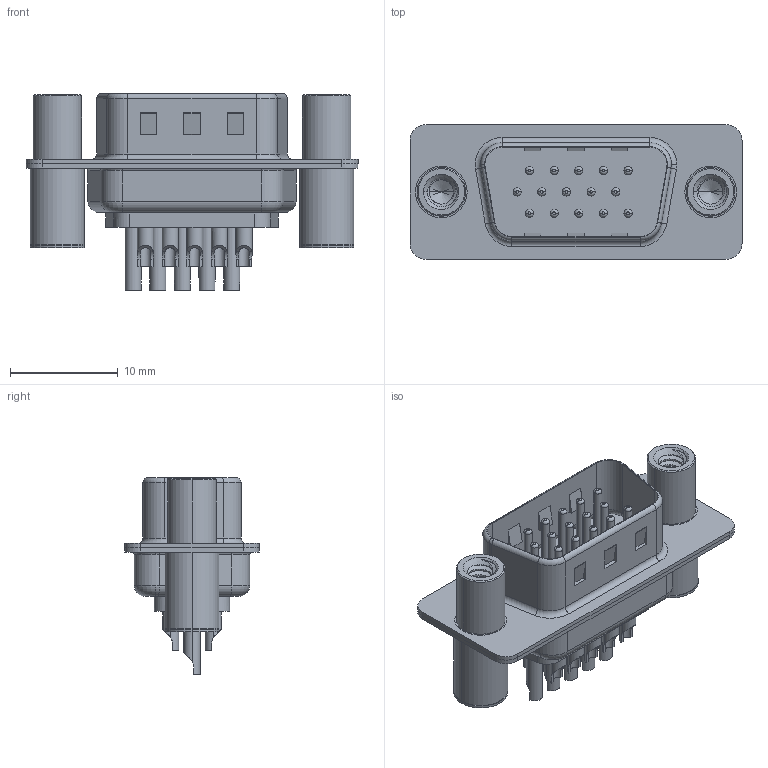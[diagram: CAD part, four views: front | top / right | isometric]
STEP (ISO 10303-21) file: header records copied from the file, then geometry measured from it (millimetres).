
FILE_DESCRIPTION (( 'STEP AP203' ), '1' );
FILE_NAME ('637-M15-232-BN4.STEP', '2018-11-19T22:10:51', ( '' ), ( '' ), 'SwSTEP 2.0', 'SolidWorks 2016', '' );
FILE_SCHEMA (( 'CONFIG_CONTROL_DESIGN' ));
Length unit declared in the file: millimetre
Products named in the file (8): 637M Contact Row 3_32; 637M 4-40 Threaded Standoff and Board Spacer; 637-M15-232-BN4; 637M Housing_15 Contacts; 637M Shell Front_15 Contacts; 637M Shell Rear_15 Contacts; 637M Contact Row 1_32; 637M Contact Row 2_32
Assembly tree (20 placements, depth 2):
  637-M15-232-BN4
    637M Housing_15 Contacts
    637M Shell Front_15 Contacts
    637M Shell Rear_15 Contacts
    637M Contact Row 1_32  x5
    637M Contact Row 2_32  x5
    637M Contact Row 3_32  x5
    637M 4-40 Threaded Standoff and Board Spacer  x2
Bounding box: 30.8 x 12.5 x 18.25 mm (x, y, z)
Volume: 1685.4 mm3; surface area: 4804.5 mm2
Topology: 20 solids, 20 shells, 945 faces, 2243 edges, 1377 vertices
Faces by surface type: cylinder 421, plane 248, torus 204, cone 60, bspline 12
Entity records: 18588 total; most frequent: CARTESIAN_POINT 4978, DIRECTION 2766, ORIENTED_EDGE 2494, EDGE_CURVE 1247, AXIS2_PLACEMENT_3D 1111, VERTEX_POINT 788, EDGE_LOOP 623, CIRCLE 573
